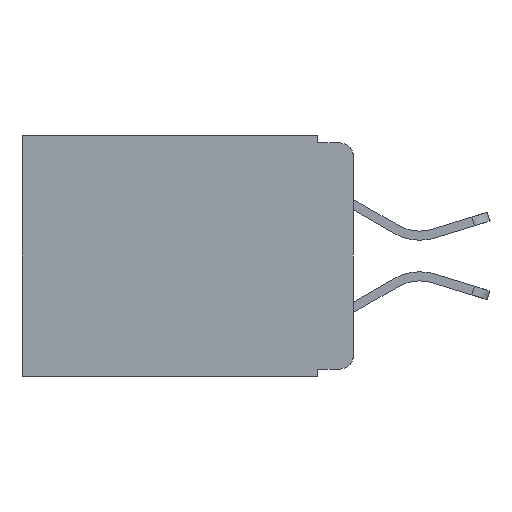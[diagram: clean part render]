
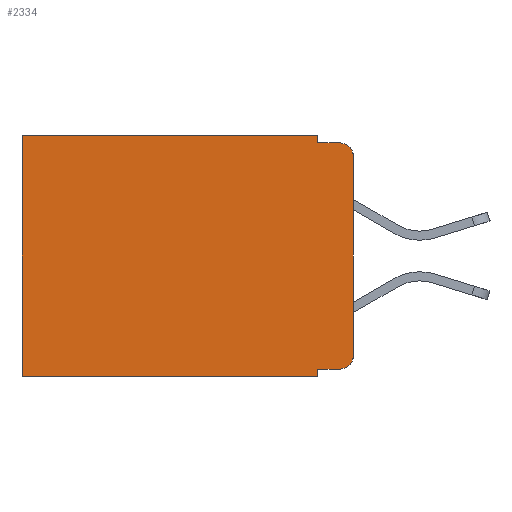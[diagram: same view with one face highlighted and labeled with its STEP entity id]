
A CAD part, left-side view. The second image highlights one B-rep face of the part: STEP entity #2334.
In plain terms, the highlighted planar face has unit normal (-1, 0, 0).
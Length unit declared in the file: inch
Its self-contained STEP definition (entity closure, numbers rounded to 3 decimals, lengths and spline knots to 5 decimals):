
#149 = VECTOR ( 'NONE', #6189, 39.37008 ) ;
#388 = EDGE_CURVE ( 'NONE', #739, #21286, #17009, .T. ) ;
#739 = VERTEX_POINT ( 'NONE', #15534 ) ;
#849 = CARTESIAN_POINT ( 'NONE',  ( 0.298, 0., 0. ) ) ;
#1053 = AXIS2_PLACEMENT_3D ( 'NONE', #14774, #4793, #16448 ) ;
#1360 = ORIENTED_EDGE ( 'NONE', *, *, #4261, .T. ) ;
#1617 = DIRECTION ( 'NONE',  ( 0., 1., 0. ) ) ;
#1707 = VECTOR ( 'NONE', #4708, 39.37008 ) ;
#1790 = LINE ( 'NONE', #849, #10312 ) ;
#1881 = VERTEX_POINT ( 'NONE', #7131 ) ;
#2024 = VECTOR ( 'NONE', #7611, 39.37008 ) ;
#2334 = ADVANCED_FACE ( 'NONE', ( #21114 ), #16513, .F. ) ;
#2547 = LINE ( 'NONE', #5891, #2024 ) ;
#3023 = VERTEX_POINT ( 'NONE', #7944 ) ;
#3266 = AXIS2_PLACEMENT_3D ( 'NONE', #8234, #18752, #9686 ) ;
#3330 = CARTESIAN_POINT ( 'NONE',  ( 0.298, 0., -0.343 ) ) ;
#3361 = VERTEX_POINT ( 'NONE', #18606 ) ;
#3402 = DIRECTION ( 'NONE',  ( -1., 0., 0. ) ) ;
#3554 = CIRCLE ( 'NONE', #18632, 0.02 ) ;
#4071 = ORIENTED_EDGE ( 'NONE', *, *, #388, .F. ) ;
#4261 = EDGE_CURVE ( 'NONE', #3361, #10427, #3554, .T. ) ;
#4708 = DIRECTION ( 'NONE',  ( 0., -1., 0. ) ) ;
#4793 = DIRECTION ( 'NONE',  ( -1., 0., 0. ) ) ;
#5141 = CIRCLE ( 'NONE', #1053, 0.02 ) ;
#5553 = CARTESIAN_POINT ( 'NONE',  ( 0.298, 0.473, 0. ) ) ;
#5694 = CARTESIAN_POINT ( 'NONE',  ( 0.298, 0.02, -0.333 ) ) ;
#5891 = CARTESIAN_POINT ( 'NONE',  ( 0.298, 0.473, 0. ) ) ;
#6032 = ORIENTED_EDGE ( 'NONE', *, *, #11088, .T. ) ;
#6134 = ORIENTED_EDGE ( 'NONE', *, *, #20167, .T. ) ;
#6189 = DIRECTION ( 'NONE',  ( 0., -1., 0. ) ) ;
#6227 = EDGE_LOOP ( 'NONE', ( #7003, #1360, #8704, #4071, #19382, #6032, #7479, #9290, #6134, #11545 ) ) ;
#6275 = LINE ( 'NONE', #8183, #1707 ) ;
#7003 = ORIENTED_EDGE ( 'NONE', *, *, #18983, .F. ) ;
#7131 = CARTESIAN_POINT ( 'NONE',  ( 0.298, 0.051, -0.343 ) ) ;
#7233 = LINE ( 'NONE', #9367, #12145 ) ;
#7246 = DIRECTION ( 'NONE',  ( 0., 0., -1. ) ) ;
#7479 = ORIENTED_EDGE ( 'NONE', *, *, #9104, .F. ) ;
#7611 = DIRECTION ( 'NONE',  ( 0., 0., -1. ) ) ;
#7735 = EDGE_CURVE ( 'NONE', #19611, #1881, #16770, .T. ) ;
#7944 = CARTESIAN_POINT ( 'NONE',  ( 0.298, 0.473, -0.343 ) ) ;
#7952 = CARTESIAN_POINT ( 'NONE',  ( 0.298, 0.051, 0. ) ) ;
#8019 = VECTOR ( 'NONE', #11381, 39.37008 ) ;
#8183 = CARTESIAN_POINT ( 'NONE',  ( 0.298, 0.051, -0.01 ) ) ;
#8234 = CARTESIAN_POINT ( 'NONE',  ( 0.298, 0., 0. ) ) ;
#8522 = LINE ( 'NONE', #3330, #16216 ) ;
#8592 = VERTEX_POINT ( 'NONE', #5553 ) ;
#8704 = ORIENTED_EDGE ( 'NONE', *, *, #11763, .F. ) ;
#9104 = EDGE_CURVE ( 'NONE', #1881, #3023, #8522, .T. ) ;
#9210 = VERTEX_POINT ( 'NONE', #10267 ) ;
#9290 = ORIENTED_EDGE ( 'NONE', *, *, #7735, .F. ) ;
#9293 = LINE ( 'NONE', #16113, #149 ) ;
#9367 = CARTESIAN_POINT ( 'NONE',  ( 0.298, 0., 0. ) ) ;
#9686 = DIRECTION ( 'NONE',  ( 0., 0., -1. ) ) ;
#10267 = CARTESIAN_POINT ( 'NONE',  ( 0.298, 0., -0.313 ) ) ;
#10312 = VECTOR ( 'NONE', #17628, 39.37008 ) ;
#10427 = VERTEX_POINT ( 'NONE', #15690 ) ;
#11088 = EDGE_CURVE ( 'NONE', #8592, #3023, #2547, .T. ) ;
#11381 = DIRECTION ( 'NONE',  ( 0., 0., -1. ) ) ;
#11545 = ORIENTED_EDGE ( 'NONE', *, *, #16990, .T. ) ;
#11763 = EDGE_CURVE ( 'NONE', #21286, #10427, #6275, .T. ) ;
#12145 = VECTOR ( 'NONE', #20683, 39.37008 ) ;
#13453 = CARTESIAN_POINT ( 'NONE',  ( 0.298, 0.02, -0.03 ) ) ;
#14774 = CARTESIAN_POINT ( 'NONE',  ( 0.298, 0.02, -0.313 ) ) ;
#15088 = DIRECTION ( 'NONE',  ( 0., 0., -1. ) ) ;
#15534 = CARTESIAN_POINT ( 'NONE',  ( 0.298, 0.051, 0. ) ) ;
#15690 = CARTESIAN_POINT ( 'NONE',  ( 0.298, 0.02, -0.01 ) ) ;
#16016 = VERTEX_POINT ( 'NONE', #5694 ) ;
#16113 = CARTESIAN_POINT ( 'NONE',  ( 0.298, 0.051, -0.333 ) ) ;
#16216 = VECTOR ( 'NONE', #1617, 39.37008 ) ;
#16305 = CARTESIAN_POINT ( 'NONE',  ( 0.298, 0.051, 0. ) ) ;
#16448 = DIRECTION ( 'NONE',  ( 0., 0., -1. ) ) ;
#16513 = PLANE ( 'NONE',  #3266 ) ;
#16770 = LINE ( 'NONE', #16305, #8019 ) ;
#16990 = EDGE_CURVE ( 'NONE', #16016, #9210, #5141, .T. ) ;
#17009 = LINE ( 'NONE', #7952, #20213 ) ;
#17628 = DIRECTION ( 'NONE',  ( 0., 1., 0. ) ) ;
#17936 = CARTESIAN_POINT ( 'NONE',  ( 0.298, 0.051, -0.333 ) ) ;
#18606 = CARTESIAN_POINT ( 'NONE',  ( 0.298, 0., -0.03 ) ) ;
#18632 = AXIS2_PLACEMENT_3D ( 'NONE', #13453, #3402, #15088 ) ;
#18752 = DIRECTION ( 'NONE',  ( 1., 0., 0. ) ) ;
#18983 = EDGE_CURVE ( 'NONE', #3361, #9210, #7233, .T. ) ;
#19382 = ORIENTED_EDGE ( 'NONE', *, *, #20128, .T. ) ;
#19611 = VERTEX_POINT ( 'NONE', #17936 ) ;
#20128 = EDGE_CURVE ( 'NONE', #739, #8592, #1790, .T. ) ;
#20167 = EDGE_CURVE ( 'NONE', #19611, #16016, #9293, .T. ) ;
#20213 = VECTOR ( 'NONE', #7246, 39.37008 ) ;
#20593 = CARTESIAN_POINT ( 'NONE',  ( 0.298, 0.051, -0.01 ) ) ;
#20683 = DIRECTION ( 'NONE',  ( 0., 0., -1. ) ) ;
#21114 = FACE_OUTER_BOUND ( 'NONE', #6227, .T. ) ;
#21286 = VERTEX_POINT ( 'NONE', #20593 ) ;
